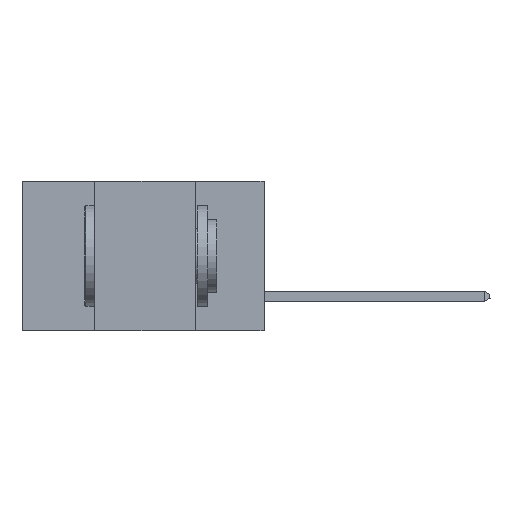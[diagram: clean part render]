
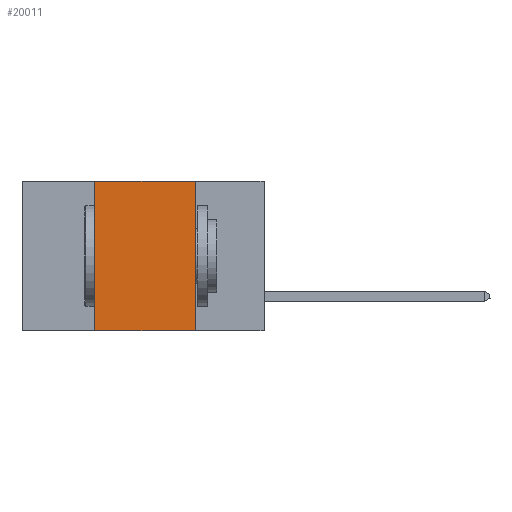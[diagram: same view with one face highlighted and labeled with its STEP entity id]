
A CAD part, left-side view. The second image highlights one B-rep face of the part: STEP entity #20011.
In plain terms, the highlighted planar face has unit normal (-1, 0, 0).
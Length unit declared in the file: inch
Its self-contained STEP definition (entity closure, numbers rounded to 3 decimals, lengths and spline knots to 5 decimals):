
#223 = VERTEX_POINT ( 'NONE', #11632 ) ;
#743 = LINE ( 'NONE', #1627, #17160 ) ;
#1031 = ORIENTED_EDGE ( 'NONE', *, *, #15656, .F. ) ;
#1545 = VERTEX_POINT ( 'NONE', #22775 ) ;
#1627 = CARTESIAN_POINT ( 'NONE',  ( 0., 0.17, 0. ) ) ;
#1683 = LINE ( 'NONE', #16940, #19180 ) ;
#3304 = LINE ( 'NONE', #5870, #6560 ) ;
#4219 = CARTESIAN_POINT ( 'NONE',  ( 0., 0.6, 0. ) ) ;
#5298 = DIRECTION ( 'NONE',  ( 0., -1., 0. ) ) ;
#5692 = EDGE_CURVE ( 'NONE', #27542, #1545, #18122, .T. ) ;
#5870 = CARTESIAN_POINT ( 'NONE',  ( 0., 0.42, 0. ) ) ;
#6169 = ORIENTED_EDGE ( 'NONE', *, *, #18448, .T. ) ;
#6370 = DIRECTION ( 'NONE',  ( 0., 0., -1. ) ) ;
#6560 = VECTOR ( 'NONE', #14965, 39.37008 ) ;
#9022 = VECTOR ( 'NONE', #15965, 39.37008 ) ;
#11632 = CARTESIAN_POINT ( 'NONE',  ( 0., 0.42, -0.37 ) ) ;
#13333 = CARTESIAN_POINT ( 'NONE',  ( 0., 0.6, 0. ) ) ;
#14213 = VERTEX_POINT ( 'NONE', #18859 ) ;
#14965 = DIRECTION ( 'NONE',  ( 0., 0., 1. ) ) ;
#15066 = EDGE_LOOP ( 'NONE', ( #1031, #22072, #25017, #6169 ) ) ;
#15656 = EDGE_CURVE ( 'NONE', #1545, #14213, #743, .T. ) ;
#15855 = FACE_OUTER_BOUND ( 'NONE', #15066, .T. ) ;
#15965 = DIRECTION ( 'NONE',  ( 0., -1., 0. ) ) ;
#16940 = CARTESIAN_POINT ( 'NONE',  ( 0., 0.6, -0.37 ) ) ;
#17160 = VECTOR ( 'NONE', #29442, 39.37008 ) ;
#18122 = LINE ( 'NONE', #4219, #9022 ) ;
#18448 = EDGE_CURVE ( 'NONE', #223, #14213, #1683, .T. ) ;
#18859 = CARTESIAN_POINT ( 'NONE',  ( 0., 0.17, -0.37 ) ) ;
#18943 = CARTESIAN_POINT ( 'NONE',  ( 0., 0.42, 0. ) ) ;
#19180 = VECTOR ( 'NONE', #5298, 39.37008 ) ;
#20011 = ADVANCED_FACE ( 'NONE', ( #15855 ), #27214, .F. ) ;
#21653 = AXIS2_PLACEMENT_3D ( 'NONE', #13333, #24735, #6370 ) ;
#21833 = EDGE_CURVE ( 'NONE', #223, #27542, #3304, .T. ) ;
#22072 = ORIENTED_EDGE ( 'NONE', *, *, #5692, .F. ) ;
#22775 = CARTESIAN_POINT ( 'NONE',  ( 0., 0.17, 0. ) ) ;
#24735 = DIRECTION ( 'NONE',  ( 1., 0., 0. ) ) ;
#25017 = ORIENTED_EDGE ( 'NONE', *, *, #21833, .F. ) ;
#27214 = PLANE ( 'NONE',  #21653 ) ;
#27542 = VERTEX_POINT ( 'NONE', #18943 ) ;
#29442 = DIRECTION ( 'NONE',  ( 0., 0., -1. ) ) ;
